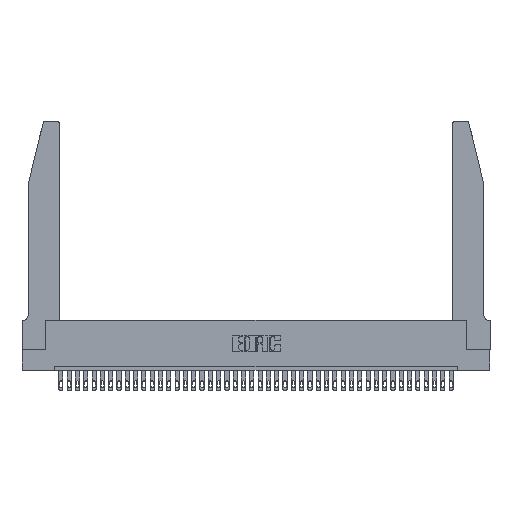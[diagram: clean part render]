
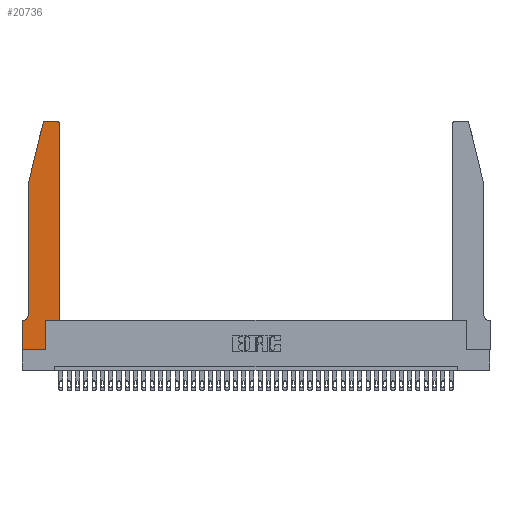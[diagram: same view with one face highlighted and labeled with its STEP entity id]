
A CAD part, top view. The second image highlights one B-rep face of the part: STEP entity #20736.
In plain terms, the highlighted planar face has unit normal (0, 0, 1).
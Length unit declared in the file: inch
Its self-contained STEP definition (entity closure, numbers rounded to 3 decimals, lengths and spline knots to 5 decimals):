
#118 = VECTOR ( 'NONE', #16382, 39.37008 ) ;
#278 = LINE ( 'NONE', #25462, #17745 ) ;
#1314 = AXIS2_PLACEMENT_3D ( 'NONE', #17936, #36588, #2563 ) ;
#2563 = DIRECTION ( 'NONE',  ( 1., 0., 0. ) ) ;
#3842 = FACE_OUTER_BOUND ( 'NONE', #17337, .T. ) ;
#4379 = EDGE_CURVE ( 'NONE', #7996, #34660, #15597, .T. ) ;
#4984 = EDGE_CURVE ( 'NONE', #15724, #17413, #11248, .T. ) ;
#5237 = CARTESIAN_POINT ( 'NONE',  ( 0.4505, 2.72, 0.37 ) ) ;
#5801 = VECTOR ( 'NONE', #30120, 39.37008 ) ;
#6475 = DIRECTION ( 'NONE',  ( 1., 0., 0. ) ) ;
#6822 = CARTESIAN_POINT ( 'NONE',  ( 0.2865, 0.35, 0.37 ) ) ;
#7325 = CARTESIAN_POINT ( 'NONE',  ( 0.0055, 0.42, 0.37 ) ) ;
#7775 = CARTESIAN_POINT ( 'NONE',  ( 0., 0.35, 0.37 ) ) ;
#7996 = VERTEX_POINT ( 'NONE', #18906 ) ;
#8331 = DIRECTION ( 'NONE',  ( 0., 0., 1. ) ) ;
#8470 = CARTESIAN_POINT ( 'NONE',  ( 0.2865, 0., 0.37 ) ) ;
#9285 = ORIENTED_EDGE ( 'NONE', *, *, #15839, .T. ) ;
#9633 = LINE ( 'NONE', #16842, #31329 ) ;
#10026 = EDGE_CURVE ( 'NONE', #18471, #38775, #36013, .T. ) ;
#11248 = CIRCLE ( 'NONE', #15103, 0.07 ) ;
#11481 = DIRECTION ( 'NONE',  ( 0., 1., 0. ) ) ;
#11617 = ORIENTED_EDGE ( 'NONE', *, *, #16383, .T. ) ;
#12256 = LINE ( 'NONE', #25955, #118 ) ;
#12918 = ORIENTED_EDGE ( 'NONE', *, *, #18459, .T. ) ;
#13264 = DIRECTION ( 'NONE',  ( 0., 0., 1. ) ) ;
#13319 = EDGE_CURVE ( 'NONE', #38775, #13819, #38102, .T. ) ;
#13819 = VERTEX_POINT ( 'NONE', #25279 ) ;
#13911 = CARTESIAN_POINT ( 'NONE',  ( 0., 0., 0.37 ) ) ;
#14449 = CARTESIAN_POINT ( 'NONE',  ( 0., 0.35, 0.37 ) ) ;
#14589 = CARTESIAN_POINT ( 'NONE',  ( 0.0755, 2., 0.37 ) ) ;
#14593 = DIRECTION ( 'NONE',  ( 1., 0., 0. ) ) ;
#15103 = AXIS2_PLACEMENT_3D ( 'NONE', #7325, #29030, #19319 ) ;
#15597 = LINE ( 'NONE', #23761, #26737 ) ;
#15724 = VERTEX_POINT ( 'NONE', #34957 ) ;
#15839 = EDGE_CURVE ( 'NONE', #18798, #7996, #17301, .T. ) ;
#16067 = CARTESIAN_POINT ( 'NONE',  ( 0.4205, 2.72, 0.37 ) ) ;
#16355 = ORIENTED_EDGE ( 'NONE', *, *, #26212, .T. ) ;
#16382 = DIRECTION ( 'NONE',  ( -0.239, -0.971, 0. ) ) ;
#16383 = EDGE_CURVE ( 'NONE', #18352, #31453, #278, .T. ) ;
#16478 = ORIENTED_EDGE ( 'NONE', *, *, #26760, .T. ) ;
#16563 = AXIS2_PLACEMENT_3D ( 'NONE', #7775, #8331, #36121 ) ;
#16842 = CARTESIAN_POINT ( 'NONE',  ( 0.2865, 0.35, 0.37 ) ) ;
#17263 = EDGE_CURVE ( 'NONE', #21209, #15724, #24862, .T. ) ;
#17301 = LINE ( 'NONE', #13911, #33232 ) ;
#17337 = EDGE_LOOP ( 'NONE', ( #28552, #31366, #12918, #39285, #31657, #34750, #9285, #34646, #29398, #16355, #11617, #16478 ) ) ;
#17413 = VERTEX_POINT ( 'NONE', #28435 ) ;
#17745 = VECTOR ( 'NONE', #37614, 39.37008 ) ;
#17936 = CARTESIAN_POINT ( 'NONE',  ( 0.284, 2.72, 0.37 ) ) ;
#18352 = VERTEX_POINT ( 'NONE', #29251 ) ;
#18459 = EDGE_CURVE ( 'NONE', #13819, #21209, #12256, .T. ) ;
#18471 = VERTEX_POINT ( 'NONE', #19514 ) ;
#18798 = VERTEX_POINT ( 'NONE', #14449 ) ;
#18906 = CARTESIAN_POINT ( 'NONE',  ( 0., 0., 0.37 ) ) ;
#19319 = DIRECTION ( 'NONE',  ( -1., 0., 0. ) ) ;
#19328 = DIRECTION ( 'NONE',  ( 1., 0., 0. ) ) ;
#19514 = CARTESIAN_POINT ( 'NONE',  ( 0.4205, 2.75, 0.37 ) ) ;
#20058 = PLANE ( 'NONE',  #16563 ) ;
#20523 = EDGE_CURVE ( 'NONE', #34660, #23359, #9633, .T. ) ;
#20736 = ADVANCED_FACE ( 'NONE', ( #3842 ), #20058, .T. ) ;
#21209 = VERTEX_POINT ( 'NONE', #22200 ) ;
#22200 = CARTESIAN_POINT ( 'NONE',  ( 0.0755, 2., 0.37 ) ) ;
#23220 = DIRECTION ( 'NONE',  ( 0., -1., 0. ) ) ;
#23359 = VERTEX_POINT ( 'NONE', #6822 ) ;
#23761 = CARTESIAN_POINT ( 'NONE',  ( 0., 0., 0.37 ) ) ;
#23894 = CARTESIAN_POINT ( 'NONE',  ( 0.0755, 0.35, 0.37 ) ) ;
#24670 = CIRCLE ( 'NONE', #29924, 0.03 ) ;
#24862 = LINE ( 'NONE', #14589, #35021 ) ;
#25279 = CARTESIAN_POINT ( 'NONE',  ( 0.25487, 2.72718, 0.37 ) ) ;
#25462 = CARTESIAN_POINT ( 'NONE',  ( 0.4505, 0.35, 0.37 ) ) ;
#25955 = CARTESIAN_POINT ( 'NONE',  ( 0.0755, 2., 0.37 ) ) ;
#26212 = EDGE_CURVE ( 'NONE', #23359, #18352, #37699, .T. ) ;
#26737 = VECTOR ( 'NONE', #14593, 39.37008 ) ;
#26739 = DIRECTION ( 'NONE',  ( -1., 0., 0. ) ) ;
#26760 = EDGE_CURVE ( 'NONE', #31453, #18471, #24670, .T. ) ;
#26876 = CARTESIAN_POINT ( 'NONE',  ( 0.2605, 2.75, 0.37 ) ) ;
#28435 = CARTESIAN_POINT ( 'NONE',  ( 0.0055, 0.35, 0.37 ) ) ;
#28552 = ORIENTED_EDGE ( 'NONE', *, *, #10026, .T. ) ;
#29030 = DIRECTION ( 'NONE',  ( 0., 0., -1. ) ) ;
#29251 = CARTESIAN_POINT ( 'NONE',  ( 0.4505, 0.35, 0.37 ) ) ;
#29398 = ORIENTED_EDGE ( 'NONE', *, *, #20523, .T. ) ;
#29529 = VECTOR ( 'NONE', #6475, 39.37008 ) ;
#29731 = EDGE_CURVE ( 'NONE', #17413, #18798, #39097, .T. ) ;
#29924 = AXIS2_PLACEMENT_3D ( 'NONE', #16067, #13264, #19328 ) ;
#30120 = DIRECTION ( 'NONE',  ( -1., 0., 0. ) ) ;
#31329 = VECTOR ( 'NONE', #11481, 39.37008 ) ;
#31366 = ORIENTED_EDGE ( 'NONE', *, *, #13319, .T. ) ;
#31399 = CARTESIAN_POINT ( 'NONE',  ( 0.4505, 0.35, 0.37 ) ) ;
#31453 = VERTEX_POINT ( 'NONE', #5237 ) ;
#31657 = ORIENTED_EDGE ( 'NONE', *, *, #4984, .T. ) ;
#32002 = CARTESIAN_POINT ( 'NONE',  ( 0.284, 2.75, 0.37 ) ) ;
#33232 = VECTOR ( 'NONE', #23220, 39.37008 ) ;
#34646 = ORIENTED_EDGE ( 'NONE', *, *, #4379, .T. ) ;
#34660 = VERTEX_POINT ( 'NONE', #8470 ) ;
#34750 = ORIENTED_EDGE ( 'NONE', *, *, #29731, .T. ) ;
#34957 = CARTESIAN_POINT ( 'NONE',  ( 0.0755, 0.42, 0.37 ) ) ;
#35021 = VECTOR ( 'NONE', #39419, 39.37008 ) ;
#36013 = LINE ( 'NONE', #26876, #39355 ) ;
#36121 = DIRECTION ( 'NONE',  ( 1., 0., 0. ) ) ;
#36588 = DIRECTION ( 'NONE',  ( 0., 0., 1. ) ) ;
#37614 = DIRECTION ( 'NONE',  ( 0., 1., 0. ) ) ;
#37699 = LINE ( 'NONE', #31399, #29529 ) ;
#38102 = CIRCLE ( 'NONE', #1314, 0.03 ) ;
#38775 = VERTEX_POINT ( 'NONE', #32002 ) ;
#39097 = LINE ( 'NONE', #23894, #5801 ) ;
#39285 = ORIENTED_EDGE ( 'NONE', *, *, #17263, .T. ) ;
#39355 = VECTOR ( 'NONE', #26739, 39.37008 ) ;
#39419 = DIRECTION ( 'NONE',  ( 0., -1., 0. ) ) ;
